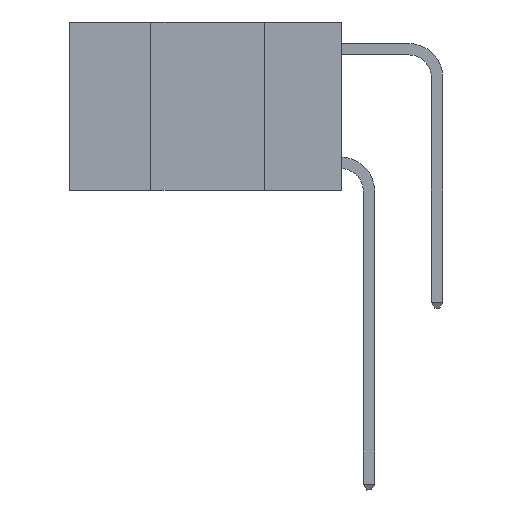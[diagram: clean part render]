
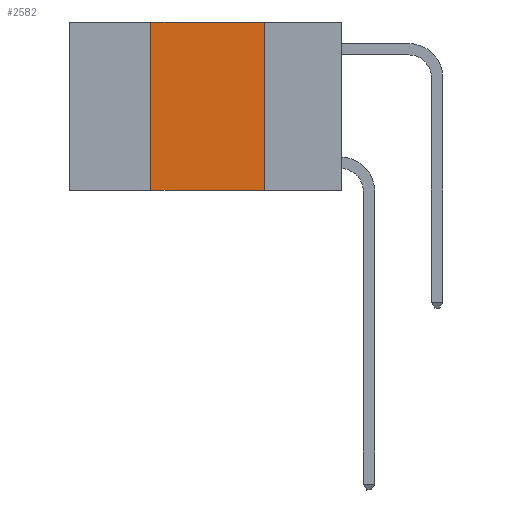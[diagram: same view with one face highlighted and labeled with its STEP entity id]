
A CAD part, left-side view. The second image highlights one B-rep face of the part: STEP entity #2582.
In plain terms, the highlighted planar face has unit normal (-1, 0, 0).
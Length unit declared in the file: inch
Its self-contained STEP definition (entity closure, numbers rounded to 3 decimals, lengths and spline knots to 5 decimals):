
#222 = ORIENTED_EDGE ( 'NONE', *, *, #613, .F. ) ;
#578 = CARTESIAN_POINT ( 'NONE',  ( 0., 0.6, 0. ) ) ;
#613 = EDGE_CURVE ( 'NONE', #10385, #2370, #6286, .T. ) ;
#715 = EDGE_LOOP ( 'NONE', ( #6716, #12694, #222, #8226 ) ) ;
#867 = VERTEX_POINT ( 'NONE', #6267 ) ;
#1860 = DIRECTION ( 'NONE',  ( 0., 0., 1. ) ) ;
#2041 = VERTEX_POINT ( 'NONE', #9825 ) ;
#2370 = VERTEX_POINT ( 'NONE', #2634 ) ;
#2582 = ADVANCED_FACE ( 'NONE', ( #4703 ), #4998, .F. ) ;
#2634 = CARTESIAN_POINT ( 'NONE',  ( 0., 0.42, 0. ) ) ;
#3145 = VECTOR ( 'NONE', #5739, 39.37008 ) ;
#3203 = CARTESIAN_POINT ( 'NONE',  ( 0., 0.42, -0.37 ) ) ;
#4360 = AXIS2_PLACEMENT_3D ( 'NONE', #7864, #11747, #5978 ) ;
#4660 = EDGE_CURVE ( 'NONE', #867, #2041, #11309, .T. ) ;
#4703 = FACE_OUTER_BOUND ( 'NONE', #715, .T. ) ;
#4765 = CARTESIAN_POINT ( 'NONE',  ( 0., 0.6, -0.37 ) ) ;
#4998 = PLANE ( 'NONE',  #4360 ) ;
#5414 = EDGE_CURVE ( 'NONE', #2370, #867, #7662, .T. ) ;
#5504 = CARTESIAN_POINT ( 'NONE',  ( 0., 0.17, 0. ) ) ;
#5567 = VECTOR ( 'NONE', #11289, 39.37008 ) ;
#5739 = DIRECTION ( 'NONE',  ( 0., -1., 0. ) ) ;
#5978 = DIRECTION ( 'NONE',  ( 0., 0., -1. ) ) ;
#6267 = CARTESIAN_POINT ( 'NONE',  ( 0., 0.17, 0. ) ) ;
#6286 = LINE ( 'NONE', #8799, #11105 ) ;
#6433 = LINE ( 'NONE', #4765, #3145 ) ;
#6716 = ORIENTED_EDGE ( 'NONE', *, *, #4660, .F. ) ;
#7662 = LINE ( 'NONE', #578, #12446 ) ;
#7864 = CARTESIAN_POINT ( 'NONE',  ( 0., 0.6, 0. ) ) ;
#8226 = ORIENTED_EDGE ( 'NONE', *, *, #11231, .T. ) ;
#8799 = CARTESIAN_POINT ( 'NONE',  ( 0., 0.42, 0. ) ) ;
#9542 = DIRECTION ( 'NONE',  ( 0., -1., 0. ) ) ;
#9825 = CARTESIAN_POINT ( 'NONE',  ( 0., 0.17, -0.37 ) ) ;
#10385 = VERTEX_POINT ( 'NONE', #3203 ) ;
#11105 = VECTOR ( 'NONE', #1860, 39.37008 ) ;
#11231 = EDGE_CURVE ( 'NONE', #10385, #2041, #6433, .T. ) ;
#11289 = DIRECTION ( 'NONE',  ( 0., 0., -1. ) ) ;
#11309 = LINE ( 'NONE', #5504, #5567 ) ;
#11747 = DIRECTION ( 'NONE',  ( 1., 0., 0. ) ) ;
#12446 = VECTOR ( 'NONE', #9542, 39.37008 ) ;
#12694 = ORIENTED_EDGE ( 'NONE', *, *, #5414, .F. ) ;
